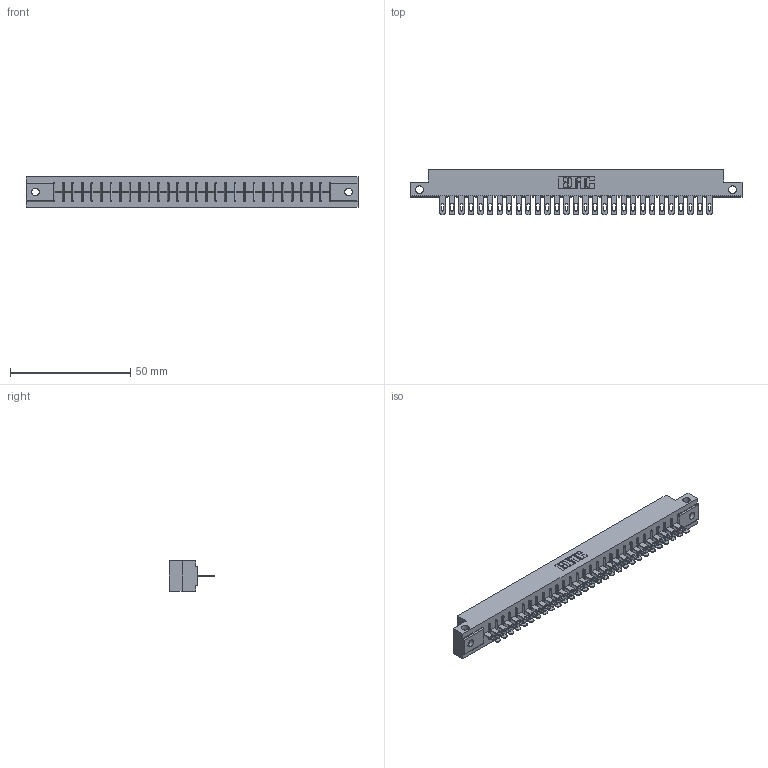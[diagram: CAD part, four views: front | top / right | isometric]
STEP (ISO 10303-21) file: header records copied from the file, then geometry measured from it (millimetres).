
FILE_DESCRIPTION (( 'STEP AP203' ), '1' );
FILE_NAME ('306-029-500-112.STEP', '2020-09-20T19:44:09', ( '' ), ( '' ), 'SwSTEP 2.0', 'SolidWorks 2020', '' );
FILE_SCHEMA (( 'CONFIG_CONTROL_DESIGN' ));
Length unit declared in the file: inch
Products named in the file (3): 306-290-001_100; 306-029-500-112; 306 Part_.128 Dia
Assembly tree (30 placements, depth 2):
  306-029-500-112
    306 Part_.128 Dia
    306-290-001_100  x29
Bounding box: 137.92 x 18.87 x 12.7 mm (x, y, z)
Volume: 15022.4 mm3; surface area: 15828.4 mm2
Topology: 30 solids, 30 shells, 2332 faces, 6587 edges, 4230 vertices
Faces by surface type: plane 1518, cylinder 698, sphere 116
Entity records: 29298 total; most frequent: CARTESIAN_POINT 4966, ORIENTED_EDGE 4878, DIRECTION 4837, EDGE_CURVE 2439, LINE 1883, VECTOR 1883, VERTEX_POINT 1542, AXIS2_PLACEMENT_3D 1477
